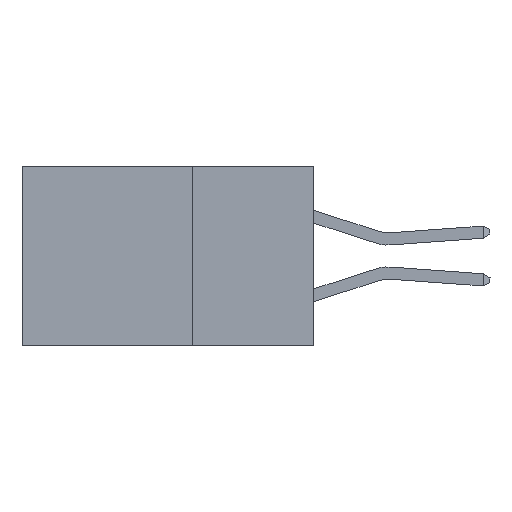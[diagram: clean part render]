
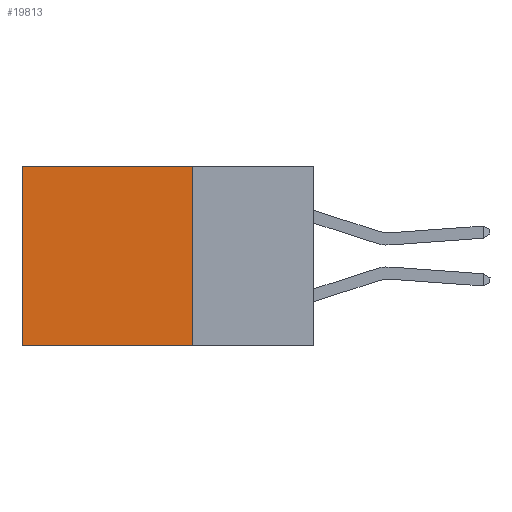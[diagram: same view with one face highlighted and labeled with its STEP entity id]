
A CAD part, left-side view. The second image highlights one B-rep face of the part: STEP entity #19813.
In plain terms, the highlighted planar face has unit normal (-1, 0, 0).
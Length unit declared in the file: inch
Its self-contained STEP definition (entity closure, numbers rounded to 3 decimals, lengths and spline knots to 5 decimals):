
#913 = LINE ( 'NONE', #9332, #23774 ) ;
#1154 = ORIENTED_EDGE ( 'NONE', *, *, #24000, .F. ) ;
#1740 = CARTESIAN_POINT ( 'NONE',  ( 0.2875, 0.25, -0.37 ) ) ;
#4039 = EDGE_CURVE ( 'NONE', #30944, #33062, #18362, .T. ) ;
#5518 = CARTESIAN_POINT ( 'NONE',  ( 0.2875, 0.25, 0. ) ) ;
#7385 = ORIENTED_EDGE ( 'NONE', *, *, #4039, .T. ) ;
#7573 = PLANE ( 'NONE',  #9158 ) ;
#7637 = CARTESIAN_POINT ( 'NONE',  ( 0.2875, 0.25, 0. ) ) ;
#7971 = VECTOR ( 'NONE', #10022, 39.37008 ) ;
#9158 = AXIS2_PLACEMENT_3D ( 'NONE', #12846, #10216, #20738 ) ;
#9332 = CARTESIAN_POINT ( 'NONE',  ( 0.2875, 0.25, 0. ) ) ;
#10008 = VERTEX_POINT ( 'NONE', #10698 ) ;
#10022 = DIRECTION ( 'NONE',  ( 0., 0., -1. ) ) ;
#10216 = DIRECTION ( 'NONE',  ( 1., 0., 0. ) ) ;
#10698 = CARTESIAN_POINT ( 'NONE',  ( 0.2875, 0.6, -0.37 ) ) ;
#10963 = DIRECTION ( 'NONE',  ( 0., 1., 0. ) ) ;
#10964 = VECTOR ( 'NONE', #23701, 39.37008 ) ;
#12846 = CARTESIAN_POINT ( 'NONE',  ( 0.2875, 0.25, 0. ) ) ;
#17246 = DIRECTION ( 'NONE',  ( 0., 0., -1. ) ) ;
#17628 = CARTESIAN_POINT ( 'NONE',  ( 0.2875, 0.25, -0.37 ) ) ;
#17933 = LINE ( 'NONE', #20722, #7971 ) ;
#18362 = LINE ( 'NONE', #5518, #20096 ) ;
#19813 = ADVANCED_FACE ( 'NONE', ( #34518 ), #7573, .F. ) ;
#19855 = CARTESIAN_POINT ( 'NONE',  ( 0.2875, 0.6, 0. ) ) ;
#20096 = VECTOR ( 'NONE', #10963, 39.37008 ) ;
#20722 = CARTESIAN_POINT ( 'NONE',  ( 0.2875, 0.6, 0. ) ) ;
#20738 = DIRECTION ( 'NONE',  ( 0., 0., -1. ) ) ;
#21993 = EDGE_CURVE ( 'NONE', #30944, #31431, #913, .T. ) ;
#22409 = ORIENTED_EDGE ( 'NONE', *, *, #33210, .T. ) ;
#23701 = DIRECTION ( 'NONE',  ( 0., 1., 0. ) ) ;
#23774 = VECTOR ( 'NONE', #17246, 39.37008 ) ;
#24000 = EDGE_CURVE ( 'NONE', #31431, #10008, #31833, .T. ) ;
#24808 = EDGE_LOOP ( 'NONE', ( #22409, #1154, #33854, #7385 ) ) ;
#30944 = VERTEX_POINT ( 'NONE', #7637 ) ;
#31431 = VERTEX_POINT ( 'NONE', #17628 ) ;
#31833 = LINE ( 'NONE', #1740, #10964 ) ;
#33062 = VERTEX_POINT ( 'NONE', #19855 ) ;
#33210 = EDGE_CURVE ( 'NONE', #33062, #10008, #17933, .T. ) ;
#33854 = ORIENTED_EDGE ( 'NONE', *, *, #21993, .F. ) ;
#34518 = FACE_OUTER_BOUND ( 'NONE', #24808, .T. ) ;
